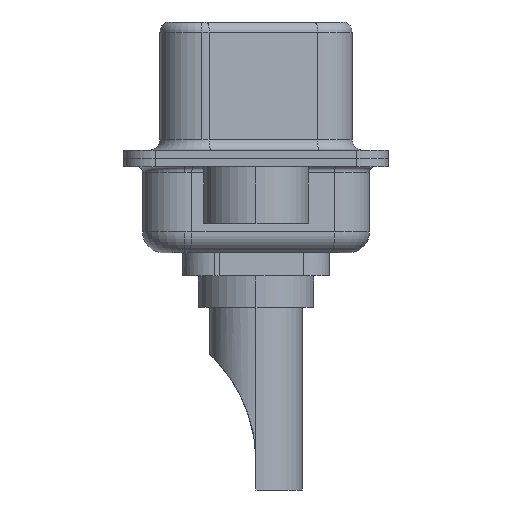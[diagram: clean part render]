
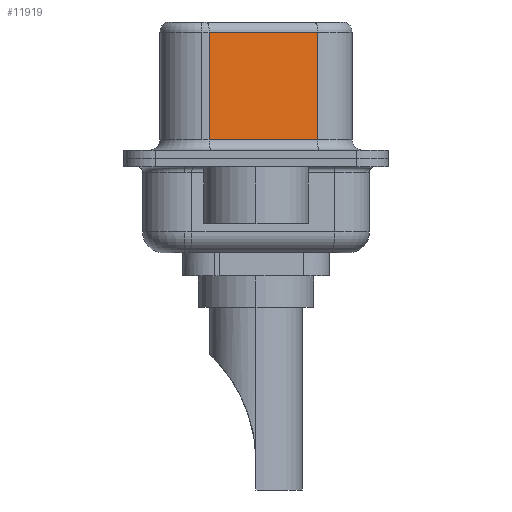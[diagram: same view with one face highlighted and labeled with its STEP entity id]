
A CAD part, left-side view. The second image highlights one B-rep face of the part: STEP entity #11919.
In plain terms, the highlighted planar face has unit normal (-0.985, -0.174, 0).
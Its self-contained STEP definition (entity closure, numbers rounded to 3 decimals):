
#1001 = DIRECTION ( 'NONE',  ( 0., 0., -1. ) ) ;
#1302 = DIRECTION ( 'NONE',  ( 0.174, -0.985, 0. ) ) ;
#1793 = ORIENTED_EDGE ( 'NONE', *, *, #13403, .T. ) ;
#2690 = LINE ( 'NONE', #17130, #3539 ) ;
#2840 = DIRECTION ( 'NONE',  ( -0.174, 0.985, 0. ) ) ;
#3539 = VECTOR ( 'NONE', #1001, 1000. ) ;
#3662 = CARTESIAN_POINT ( 'NONE',  ( 3.675, 2.233, 6.02 ) ) ;
#3835 = VECTOR ( 'NONE', #6423, 1000. ) ;
#4318 = ORIENTED_EDGE ( 'NONE', *, *, #6054, .F. ) ;
#4681 = ORIENTED_EDGE ( 'NONE', *, *, #7909, .T. ) ;
#5801 = EDGE_LOOP ( 'NONE', ( #4318, #14362, #1793, #4681 ) ) ;
#6054 = EDGE_CURVE ( 'NONE', #9099, #8082, #7391, .T. ) ;
#6423 = DIRECTION ( 'NONE',  ( 0., 0., -1. ) ) ;
#6479 = VECTOR ( 'NONE', #1302, 1000. ) ;
#6512 = DIRECTION ( 'NONE',  ( -0.174, 0.985, 0. ) ) ;
#6656 = LINE ( 'NONE', #10556, #13369 ) ;
#6921 = FACE_OUTER_BOUND ( 'NONE', #5801, .T. ) ;
#7356 = LINE ( 'NONE', #13444, #6479 ) ;
#7391 = LINE ( 'NONE', #9061, #3835 ) ;
#7909 = EDGE_CURVE ( 'NONE', #12798, #8082, #7356, .T. ) ;
#8082 = VERTEX_POINT ( 'NONE', #8516 ) ;
#8209 = PLANE ( 'NONE',  #16045 ) ;
#8516 = CARTESIAN_POINT ( 'NONE',  ( 4.585, -2.927, 0.9 ) ) ;
#9061 = CARTESIAN_POINT ( 'NONE',  ( 4.585, -2.927, 6.52 ) ) ;
#9099 = VERTEX_POINT ( 'NONE', #12443 ) ;
#10527 = CARTESIAN_POINT ( 'NONE',  ( 3.675, 2.233, 0.9 ) ) ;
#10556 = CARTESIAN_POINT ( 'NONE',  ( 4.585, -2.927, 6.02 ) ) ;
#10899 = DIRECTION ( 'NONE',  ( 0.985, 0.174, 0. ) ) ;
#11919 = ADVANCED_FACE ( 'NONE', ( #6921 ), #8209, .F. ) ;
#12443 = CARTESIAN_POINT ( 'NONE',  ( 4.585, -2.927, 6.02 ) ) ;
#12798 = VERTEX_POINT ( 'NONE', #10527 ) ;
#13369 = VECTOR ( 'NONE', #6512, 1000. ) ;
#13403 = EDGE_CURVE ( 'NONE', #14723, #12798, #2690, .T. ) ;
#13444 = CARTESIAN_POINT ( 'NONE',  ( 4.585, -2.927, 0.9 ) ) ;
#14102 = EDGE_CURVE ( 'NONE', #9099, #14723, #6656, .T. ) ;
#14362 = ORIENTED_EDGE ( 'NONE', *, *, #14102, .T. ) ;
#14723 = VERTEX_POINT ( 'NONE', #3662 ) ;
#16045 = AXIS2_PLACEMENT_3D ( 'NONE', #17229, #10899, #2840 ) ;
#17130 = CARTESIAN_POINT ( 'NONE',  ( 3.675, 2.233, 6.52 ) ) ;
#17229 = CARTESIAN_POINT ( 'NONE',  ( 4.585, -2.927, 6.52 ) ) ;
